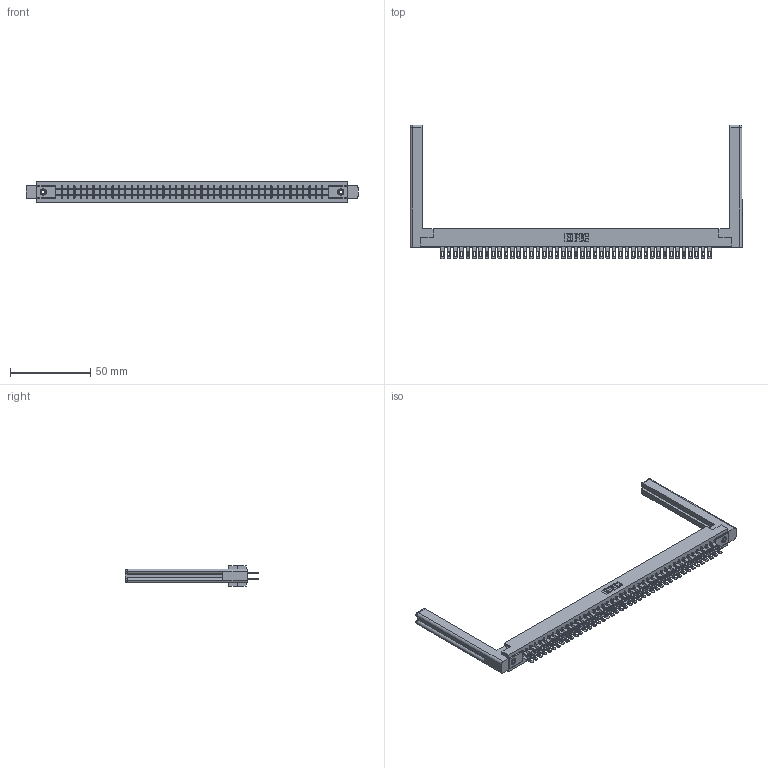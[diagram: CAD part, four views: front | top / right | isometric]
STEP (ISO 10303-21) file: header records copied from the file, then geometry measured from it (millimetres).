
FILE_DESCRIPTION (( 'STEP AP203' ), '1' );
FILE_NAME ('305-086-500-558.STEP', '2019-09-10T12:42:19', ( '' ), ( '' ), 'SwSTEP 2.0', 'SolidWorks 2016', '' );
FILE_SCHEMA (( 'CONFIG_CONTROL_DESIGN' ));
Length unit declared in the file: inch
Products named in the file (5): 305 Part_.156 Dia; 345-250-001_345-250-001-102; 305-290-001_500; 307-220-058; 305-086-500-558
Assembly tree (91 placements, depth 2):
  305-086-500-558
    305 Part_.156 Dia
    305-290-001_500  x86
    345-250-001_345-250-001-102  x2
    307-220-058  x2
Bounding box: 207.01 x 83.49 x 12.7 mm (x, y, z)
Volume: 28430.6 mm3; surface area: 34580.6 mm2
Topology: 91 solids, 91 shells, 4558 faces, 13011 edges, 8430 vertices
Faces by surface type: plane 2560, cylinder 1802, sphere 172, cone 12, torus 12
Entity records: 49091 total; most frequent: CARTESIAN_POINT 8138, ORIENTED_EDGE 8020, DIRECTION 7836, EDGE_CURVE 4010, LINE 3232, VECTOR 3232, VERTEX_POINT 2550, AXIS2_PLACEMENT_3D 2302
